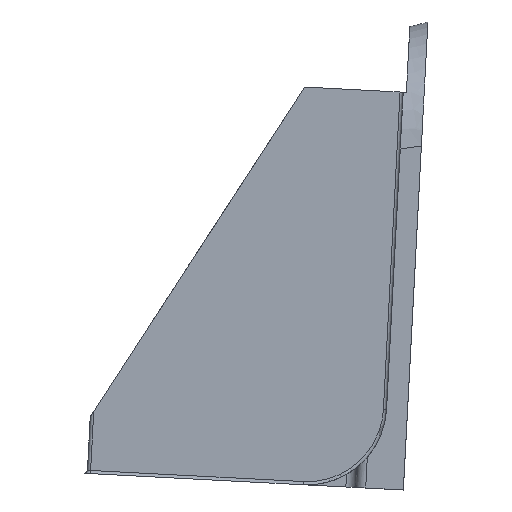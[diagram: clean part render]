
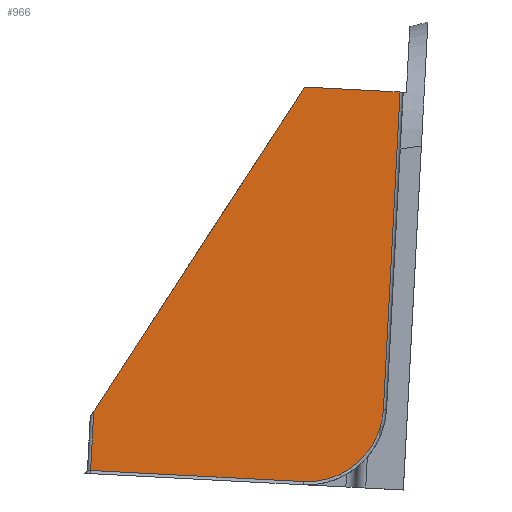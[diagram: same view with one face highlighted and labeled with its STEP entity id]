
A CAD part, left-side view. The second image highlights one B-rep face of the part: STEP entity #966.
In plain terms, the highlighted planar face has unit normal (-1, 0, 0).
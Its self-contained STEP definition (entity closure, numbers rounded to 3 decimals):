
#48 = FACE_OUTER_BOUND ( 'NONE', #469, .T. ) ;
#73 = DIRECTION ( 'NONE',  ( 0., -0.052, 0.999 ) ) ;
#82 = CARTESIAN_POINT ( 'NONE',  ( 7.953, 0.062, 2.771 ) ) ;
#87 = DIRECTION ( 'NONE',  ( 0., 0.052, -0.999 ) ) ;
#99 = AXIS2_PLACEMENT_3D ( 'NONE', #623, #609, #600 ) ;
#101 = CARTESIAN_POINT ( 'NONE',  ( 7.953, 23.144, 3.981 ) ) ;
#109 = EDGE_CURVE ( 'NONE', #1305, #978, #1751, .T. ) ;
#111 = CARTESIAN_POINT ( 'NONE',  ( 7.953, -3.984, 136.023 ) ) ;
#134 = CARTESIAN_POINT ( 'NONE',  ( 7.953, -3.801, 135.929 ) ) ;
#142 = CARTESIAN_POINT ( 'NONE',  ( 7.953, -6.724, 139.036 ) ) ;
#159 = CARTESIAN_POINT ( 'NONE',  ( 7.953, -3.524, 135.795 ) ) ;
#178 = ORIENTED_EDGE ( 'NONE', *, *, #294, .T. ) ;
#245 = CARTESIAN_POINT ( 'NONE',  ( 7.953, -3.238, 135.682 ) ) ;
#259 = CARTESIAN_POINT ( 'NONE',  ( 7.953, -2.994, 135.6 ) ) ;
#266 = CARTESIAN_POINT ( 'NONE',  ( 7.953, -2.949, 135.585 ) ) ;
#280 = CARTESIAN_POINT ( 'NONE',  ( 7.953, -2.379, 135.428 ) ) ;
#294 = EDGE_CURVE ( 'NONE', #844, #1044, #532, .T. ) ;
#297 = EDGE_CURVE ( 'NONE', #1044, #1342, #1543, .T. ) ;
#423 = CARTESIAN_POINT ( 'NONE',  ( 7.953, -6.621, 138.812 ) ) ;
#426 = VECTOR ( 'NONE', #1052, 1000. ) ;
#469 = EDGE_LOOP ( 'NONE', ( #1717, #1021, #1119, #1362, #178, #1498 ) ) ;
#507 = CARTESIAN_POINT ( 'NONE',  ( 7.953, -6.553, 138.671 ) ) ;
#514 = CARTESIAN_POINT ( 'NONE',  ( 7.953, -6.598, 138.763 ) ) ;
#532 = LINE ( 'NONE', #989, #426 ) ;
#536 = EDGE_CURVE ( 'NONE', #1342, #1562, #645, .T. ) ;
#543 = EDGE_CURVE ( 'NONE', #978, #844, #1612, .T. ) ;
#586 = CARTESIAN_POINT ( 'NONE',  ( 7.953, -7.186, 141.075 ) ) ;
#600 = DIRECTION ( 'NONE',  ( 0., 0.052, -0.999 ) ) ;
#609 = DIRECTION ( 'NONE',  ( -1., 0., 0. ) ) ;
#623 = CARTESIAN_POINT ( 'NONE',  ( 7.953, -27.218, 1.342 ) ) ;
#629 = PLANE ( 'NONE',  #99 ) ;
#645 = LINE ( 'NONE', #101, #1309 ) ;
#672 = CARTESIAN_POINT ( 'NONE',  ( 7.953, -6.483, 138.533 ) ) ;
#675 = CARTESIAN_POINT ( 'NONE',  ( 7.953, -6.31, 138.219 ) ) ;
#680 = CARTESIAN_POINT ( 'NONE',  ( 7.953, -2.855, 135.556 ) ) ;
#695 = CARTESIAN_POINT ( 'NONE',  ( 7.953, -2.713, 135.514 ) ) ;
#702 = CARTESIAN_POINT ( 'NONE',  ( 7.953, -2.088, 135.376 ) ) ;
#710 = CARTESIAN_POINT ( 'NONE',  ( 7.953, -1.868, 135.347 ) ) ;
#755 = CARTESIAN_POINT ( 'NONE',  ( 7.953, -5.893, 137.628 ) ) ;
#757 = CARTESIAN_POINT ( 'NONE',  ( 7.953, -5.989, 137.754 ) ) ;
#764 = CARTESIAN_POINT ( 'NONE',  ( 7.953, -6.141, 137.962 ) ) ;
#779 = CARTESIAN_POINT ( 'NONE',  ( 7.953, -5.957, 137.711 ) ) ;
#805 = CARTESIAN_POINT ( 'NONE',  ( 7.953, -1.846, 135.344 ) ) ;
#825 = CARTESIAN_POINT ( 'NONE',  ( 7.953, -1.8, 135.338 ) ) ;
#830 = CARTESIAN_POINT ( 'NONE',  ( 7.953, -1.731, 135.331 ) ) ;
#837 = CARTESIAN_POINT ( 'NONE',  ( 7.953, -1.569, 135.315 ) ) ;
#844 = VERTEX_POINT ( 'NONE', #1096 ) ;
#847 = CARTESIAN_POINT ( 'NONE',  ( 7.953, -0.78, 135.306 ) ) ;
#859 = CARTESIAN_POINT ( 'NONE',  ( 7.953, 16.215, 136.197 ) ) ;
#887 = CARTESIAN_POINT ( 'NONE',  ( 7.953, -34.148, 133.558 ) ) ;
#934 = VECTOR ( 'NONE', #73, 1000. ) ;
#953 = DIRECTION ( 'NONE',  ( 0., 0.545, -0.839 ) ) ;
#960 = CARTESIAN_POINT ( 'NONE',  ( 7.953, -0.878, 166.84 ) ) ;
#961 = CARTESIAN_POINT ( 'NONE',  ( 7.953, -0.966, 135.297 ) ) ;
#966 = ADVANCED_FACE ( 'NONE', ( #48 ), #629, .T. ) ;
#968 = VECTOR ( 'NONE', #1506, 1000. ) ;
#977 = CARTESIAN_POINT ( 'NONE',  ( 7.953, -1.245, 135.295 ) ) ;
#978 = VERTEX_POINT ( 'NONE', #586 ) ;
#989 = CARTESIAN_POINT ( 'NONE',  ( 7.953, -35.796, 165.01 ) ) ;
#1009 = LINE ( 'NONE', #887, #968 ) ;
#1021 = ORIENTED_EDGE ( 'NONE', *, *, #1413, .T. ) ;
#1026 = CARTESIAN_POINT ( 'NONE',  ( 7.953, 15.969, 140.898 ) ) ;
#1044 = VERTEX_POINT ( 'NONE', #1696 ) ;
#1052 = DIRECTION ( 'NONE',  ( 0., 0.999, 0.052 ) ) ;
#1096 = CARTESIAN_POINT ( 'NONE',  ( 7.953, -8.516, 166.44 ) ) ;
#1119 = ORIENTED_EDGE ( 'NONE', *, *, #109, .T. ) ;
#1161 = CARTESIAN_POINT ( 'NONE',  ( 7.953, -5.556, 137.226 ) ) ;
#1194 = CARTESIAN_POINT ( 'NONE',  ( 7.953, -5.334, 137.004 ) ) ;
#1305 = VERTEX_POINT ( 'NONE', #1410 ) ;
#1309 = VECTOR ( 'NONE', #87, 1000. ) ;
#1342 = VERTEX_POINT ( 'NONE', #1026 ) ;
#1362 = ORIENTED_EDGE ( 'NONE', *, *, #543, .T. ) ;
#1410 = CARTESIAN_POINT ( 'NONE',  ( 7.953, -0.78, 135.306 ) ) ;
#1413 = EDGE_CURVE ( 'NONE', #1562, #1305, #1009, .T. ) ;
#1464 = VECTOR ( 'NONE', #953, 1000. ) ;
#1498 = ORIENTED_EDGE ( 'NONE', *, *, #297, .T. ) ;
#1506 = DIRECTION ( 'NONE',  ( 0., -0.999, -0.052 ) ) ;
#1543 = LINE ( 'NONE', #960, #1464 ) ;
#1562 = VERTEX_POINT ( 'NONE', #859 ) ;
#1612 = LINE ( 'NONE', #82, #934 ) ;
#1626 = CARTESIAN_POINT ( 'NONE',  ( 7.953, -4.865, 136.582 ) ) ;
#1688 = CARTESIAN_POINT ( 'NONE',  ( 7.953, -4.526, 136.335 ) ) ;
#1692 = CARTESIAN_POINT ( 'NONE',  ( 7.953, -5.795, 137.505 ) ) ;
#1696 = CARTESIAN_POINT ( 'NONE',  ( 7.953, -0.878, 166.84 ) ) ;
#1716 = CARTESIAN_POINT ( 'NONE',  ( 7.953, -4.072, 136.071 ) ) ;
#1717 = ORIENTED_EDGE ( 'NONE', *, *, #536, .T. ) ;
#1723 = CARTESIAN_POINT ( 'NONE',  ( 7.953, -7.186, 141.075 ) ) ;
#1728 = CARTESIAN_POINT ( 'NONE',  ( 7.953, -7.167, 140.702 ) ) ;
#1732 = CARTESIAN_POINT ( 'NONE',  ( 7.953, -7.113, 140.335 ) ) ;
#1737 = CARTESIAN_POINT ( 'NONE',  ( 7.953, -7.021, 139.95 ) ) ;
#1740 = CARTESIAN_POINT ( 'NONE',  ( 7.953, -7.015, 139.925 ) ) ;
#1746 = CARTESIAN_POINT ( 'NONE',  ( 7.953, -7.003, 139.877 ) ) ;
#1751 = B_SPLINE_CURVE_WITH_KNOTS ( 'NONE', 3,
 ( #847, #961, #977, #837, #830, #825, #805, #710, #702, #280, #695, #680, #266, #259, #245, #159, #134, #111, #1716, #1688, #1626, #1194, #1161, #1692, #755, #779, #757, #764, #675, #672, #507, #514, #423, #142, #1765, #1758, #1752, #1746, #1740, #1737, #1732, #1728, #1723 ),
 .UNSPECIFIED., .F., .F.,
 ( 4, 1, 1, 1, 2, 2, 1, 1, 2, 2, 1, 2, 2, 2, 1, 1, 2, 2, 1, 1, 2, 2, 1, 1, 1, 2, 2, 4 ),
 ( 0., 0.062, 0.094, 0.109, 0.117, 0.125, 0.187, 0.219, 0.234, 0.25, 0.312, 0.344, 0.375, 0.5, 0.562, 0.594, 0.609, 0.625, 0.687, 0.719, 0.734, 0.75, 0.812, 0.844, 0.859, 0.867, 0.875, 1. ),
 .UNSPECIFIED. ) ;
#1752 = CARTESIAN_POINT ( 'NONE',  ( 7.953, -6.984, 139.805 ) ) ;
#1758 = CARTESIAN_POINT ( 'NONE',  ( 7.953, -6.938, 139.639 ) ) ;
#1765 = CARTESIAN_POINT ( 'NONE',  ( 7.953, -6.833, 139.31 ) ) ;
